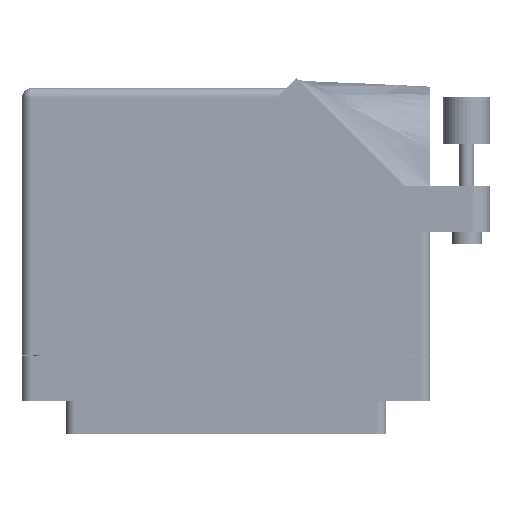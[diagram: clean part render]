
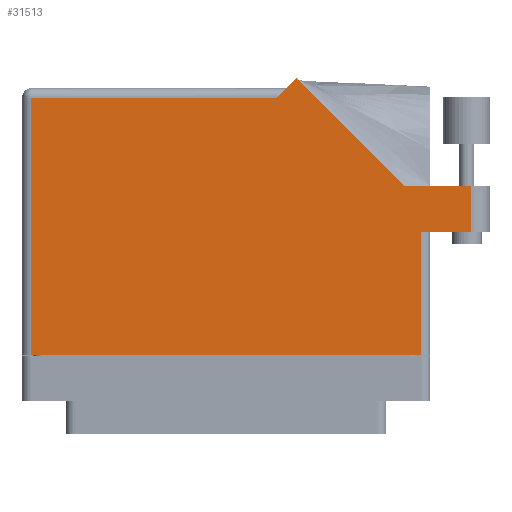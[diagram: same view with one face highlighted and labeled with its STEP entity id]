
A CAD part, front view. The second image highlights one B-rep face of the part: STEP entity #31513.
In plain terms, the highlighted face is planar.
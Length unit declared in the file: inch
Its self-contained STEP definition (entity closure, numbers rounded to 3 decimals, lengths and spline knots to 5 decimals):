
#150 = EDGE_CURVE ( 'NONE', #9776, #6696, #5523, .T. ) ;
#1012 = CARTESIAN_POINT ( 'NONE',  ( 1.19342, 1.022, 0.617 ) ) ;
#1041 = VECTOR ( 'NONE', #2777, 39.37008 ) ;
#1809 = LINE ( 'NONE', #56268, #12870 ) ;
#2587 = DIRECTION ( 'NONE',  ( 1., 0., 0. ) ) ;
#2615 = EDGE_CURVE ( 'NONE', #50619, #63846, #62962, .T. ) ;
#2777 = DIRECTION ( 'NONE',  ( 0., 1., 0. ) ) ;
#3020 = VERTEX_POINT ( 'NONE', #54285 ) ;
#3240 = DIRECTION ( 'NONE',  ( 0., -1., 0. ) ) ;
#3392 = LINE ( 'NONE', #14092, #11033 ) ;
#3736 = DIRECTION ( 'NONE',  ( 0., 1., 0. ) ) ;
#4538 = ORIENTED_EDGE ( 'NONE', *, *, #50450, .T. ) ;
#5523 = LINE ( 'NONE', #49585, #37864 ) ;
#6696 = VERTEX_POINT ( 'NONE', #51482 ) ;
#9776 = VERTEX_POINT ( 'NONE', #54303 ) ;
#9894 = CARTESIAN_POINT ( 'NONE',  ( 1.297, -0.1, 0.617 ) ) ;
#10605 = VERTEX_POINT ( 'NONE', #26960 ) ;
#11033 = VECTOR ( 'NONE', #57460, 39.37008 ) ;
#12537 = CARTESIAN_POINT ( 'NONE',  ( 1.297, 0.715, 0.617 ) ) ;
#12870 = VECTOR ( 'NONE', #2587, 39.37008 ) ;
#14092 = CARTESIAN_POINT ( 'NONE',  ( -1.359, -0.1, 0.617 ) ) ;
#14704 = LINE ( 'NONE', #36770, #57057 ) ;
#14941 = LINE ( 'NONE', #1012, #54774 ) ;
#15480 = VERTEX_POINT ( 'NONE', #12537 ) ;
#15516 = LINE ( 'NONE', #67877, #1041 ) ;
#16529 = VECTOR ( 'NONE', #38647, 39.37008 ) ;
#16556 = EDGE_CURVE ( 'NONE', #28211, #9776, #14941, .T. ) ;
#17028 = CARTESIAN_POINT ( 'NONE',  ( 1.759, 1.022, 0.617 ) ) ;
#17111 = DIRECTION ( 'NONE',  ( -0.707, -0.707, 0. ) ) ;
#21454 = EDGE_CURVE ( 'NONE', #6696, #50619, #63701, .T. ) ;
#22393 = ORIENTED_EDGE ( 'NONE', *, *, #2615, .T. ) ;
#22433 = CARTESIAN_POINT ( 'NONE',  ( -1.359, 1.675, 0.617 ) ) ;
#23864 = VERTEX_POINT ( 'NONE', #9894 ) ;
#26955 = CARTESIAN_POINT ( 'NONE',  ( -1.297, 1.613, 0.617 ) ) ;
#26960 = CARTESIAN_POINT ( 'NONE',  ( 1.634, 1.022, 0.617 ) ) ;
#27235 = EDGE_LOOP ( 'NONE', ( #38499, #4538, #27554, #47640, #48787, #43539, #22393, #59179, #61274 ) ) ;
#27554 = ORIENTED_EDGE ( 'NONE', *, *, #47201, .T. ) ;
#27830 = CARTESIAN_POINT ( 'NONE',  ( 1.19342, 1.022, 0.617 ) ) ;
#28211 = VERTEX_POINT ( 'NONE', #27830 ) ;
#31513 = ADVANCED_FACE ( 'NONE', ( #60308 ), #33352, .F. ) ;
#31940 = CARTESIAN_POINT ( 'NONE',  ( -1.297, -0.1, 0.617 ) ) ;
#32842 = DIRECTION ( 'NONE',  ( -1., 0., 0. ) ) ;
#33352 = PLANE ( 'NONE',  #60289 ) ;
#36574 = VECTOR ( 'NONE', #32842, 39.37008 ) ;
#36770 = CARTESIAN_POINT ( 'NONE',  ( 1.634, 1.022, 0.617 ) ) ;
#37864 = VECTOR ( 'NONE', #17111, 39.37008 ) ;
#38111 = EDGE_CURVE ( 'NONE', #15480, #3020, #1809, .T. ) ;
#38499 = ORIENTED_EDGE ( 'NONE', *, *, #38111, .T. ) ;
#38647 = DIRECTION ( 'NONE',  ( -1., 0., 0. ) ) ;
#39230 = DIRECTION ( 'NONE',  ( -0.707, 0.707, 0. ) ) ;
#43539 = ORIENTED_EDGE ( 'NONE', *, *, #21454, .T. ) ;
#47201 = EDGE_CURVE ( 'NONE', #10605, #28211, #56414, .T. ) ;
#47640 = ORIENTED_EDGE ( 'NONE', *, *, #16556, .T. ) ;
#48787 = ORIENTED_EDGE ( 'NONE', *, *, #150, .T. ) ;
#49585 = CARTESIAN_POINT ( 'NONE',  ( 0.399, 1.675, 0.617 ) ) ;
#50432 = EDGE_CURVE ( 'NONE', #23864, #15480, #15516, .T. ) ;
#50450 = EDGE_CURVE ( 'NONE', #3020, #10605, #14704, .T. ) ;
#50619 = VERTEX_POINT ( 'NONE', #26955 ) ;
#51482 = CARTESIAN_POINT ( 'NONE',  ( 0.337, 1.613, 0.617 ) ) ;
#54285 = CARTESIAN_POINT ( 'NONE',  ( 1.634, 0.715, 0.617 ) ) ;
#54303 = CARTESIAN_POINT ( 'NONE',  ( 0.46971, 1.74571, 0.617 ) ) ;
#54774 = VECTOR ( 'NONE', #39230, 39.37008 ) ;
#55382 = DIRECTION ( 'NONE',  ( 0., 0., -1. ) ) ;
#56268 = CARTESIAN_POINT ( 'NONE',  ( 1.359, 0.715, 0.617 ) ) ;
#56414 = LINE ( 'NONE', #17028, #16529 ) ;
#57020 = VECTOR ( 'NONE', #3240, 39.37008 ) ;
#57057 = VECTOR ( 'NONE', #3736, 39.37008 ) ;
#57460 = DIRECTION ( 'NONE',  ( 1., 0., 0. ) ) ;
#58958 = EDGE_CURVE ( 'NONE', #63846, #23864, #3392, .T. ) ;
#59179 = ORIENTED_EDGE ( 'NONE', *, *, #58958, .T. ) ;
#59887 = CARTESIAN_POINT ( 'NONE',  ( -1.359, 1.613, 0.617 ) ) ;
#60289 = AXIS2_PLACEMENT_3D ( 'NONE', #22433, #55382, #66096 ) ;
#60308 = FACE_OUTER_BOUND ( 'NONE', #27235, .T. ) ;
#61274 = ORIENTED_EDGE ( 'NONE', *, *, #50432, .T. ) ;
#62962 = LINE ( 'NONE', #68089, #57020 ) ;
#63701 = LINE ( 'NONE', #59887, #36574 ) ;
#63846 = VERTEX_POINT ( 'NONE', #31940 ) ;
#66096 = DIRECTION ( 'NONE',  ( -1., 0., 0. ) ) ;
#67877 = CARTESIAN_POINT ( 'NONE',  ( 1.297, 0.715, 0.617 ) ) ;
#68089 = CARTESIAN_POINT ( 'NONE',  ( -1.297, -0.1, 0.617 ) ) ;
